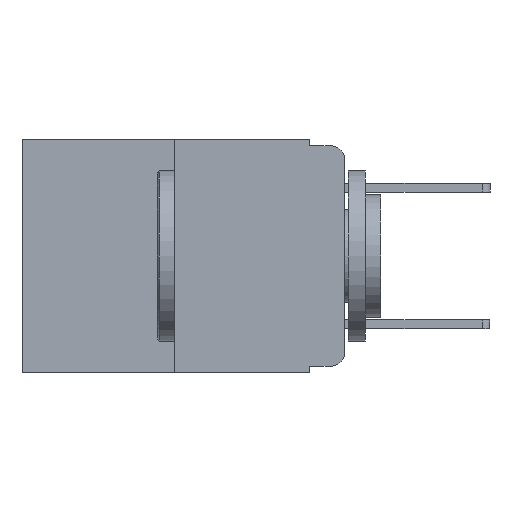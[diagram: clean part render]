
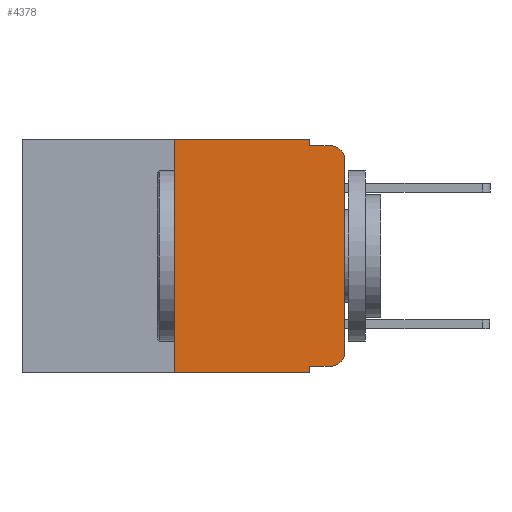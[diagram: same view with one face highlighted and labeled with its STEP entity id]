
A CAD part, left-side view. The second image highlights one B-rep face of the part: STEP entity #4378.
In plain terms, the highlighted planar face has unit normal (-1, 0, 0).
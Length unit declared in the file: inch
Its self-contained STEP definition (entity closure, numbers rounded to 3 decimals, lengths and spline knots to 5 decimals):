
#37 = DIRECTION ( 'NONE',  ( 0., 0., -1. ) ) ;
#82 = ORIENTED_EDGE ( 'NONE', *, *, #7105, .T. ) ;
#223 = LINE ( 'NONE', #6069, #14156 ) ;
#320 = ORIENTED_EDGE ( 'NONE', *, *, #5333, .T. ) ;
#467 = ORIENTED_EDGE ( 'NONE', *, *, #9116, .T. ) ;
#565 = CARTESIAN_POINT ( 'NONE',  ( 0., 0.25, 0. ) ) ;
#1006 = DIRECTION ( 'NONE',  ( 0., -1., 0. ) ) ;
#1042 = DIRECTION ( 'NONE',  ( -1., 0., 0. ) ) ;
#1183 = FACE_OUTER_BOUND ( 'NONE', #17274, .T. ) ;
#1444 = VECTOR ( 'NONE', #16356, 39.37008 ) ;
#1586 = CARTESIAN_POINT ( 'NONE',  ( 0., 0.25, 0. ) ) ;
#1604 = ORIENTED_EDGE ( 'NONE', *, *, #12360, .F. ) ;
#1745 = VERTEX_POINT ( 'NONE', #8723 ) ;
#1826 = CIRCLE ( 'NONE', #4819, 0.02 ) ;
#2852 = LINE ( 'NONE', #10554, #6090 ) ;
#3001 = DIRECTION ( 'NONE',  ( -1., 0., 0. ) ) ;
#3358 = CARTESIAN_POINT ( 'NONE',  ( 0., 0.051, -0.333 ) ) ;
#3367 = CARTESIAN_POINT ( 'NONE',  ( 0., 0.25, -0.343 ) ) ;
#3584 = LINE ( 'NONE', #8337, #10679 ) ;
#4138 = CARTESIAN_POINT ( 'NONE',  ( 0., 0., -0.313 ) ) ;
#4378 = ADVANCED_FACE ( 'NONE', ( #1183 ), #14794, .F. ) ;
#4601 = VECTOR ( 'NONE', #8008, 39.37008 ) ;
#4819 = AXIS2_PLACEMENT_3D ( 'NONE', #11004, #3001, #12320 ) ;
#4850 = VERTEX_POINT ( 'NONE', #4138 ) ;
#5333 = EDGE_CURVE ( 'NONE', #1745, #4850, #1826, .T. ) ;
#5754 = DIRECTION ( 'NONE',  ( 0., 0., -1. ) ) ;
#5773 = ORIENTED_EDGE ( 'NONE', *, *, #11507, .F. ) ;
#5962 = VERTEX_POINT ( 'NONE', #12768 ) ;
#6069 = CARTESIAN_POINT ( 'NONE',  ( 0., 0.051, -0.333 ) ) ;
#6090 = VECTOR ( 'NONE', #15634, 39.37008 ) ;
#6139 = AXIS2_PLACEMENT_3D ( 'NONE', #9271, #1042, #10580 ) ;
#6631 = CARTESIAN_POINT ( 'NONE',  ( 0., 0.473, -0.343 ) ) ;
#6642 = CARTESIAN_POINT ( 'NONE',  ( 0., 0.051, 0. ) ) ;
#6813 = ORIENTED_EDGE ( 'NONE', *, *, #13216, .T. ) ;
#7105 = EDGE_CURVE ( 'NONE', #8234, #1745, #223, .T. ) ;
#7945 = CARTESIAN_POINT ( 'NONE',  ( 0., 0.051, -0.01 ) ) ;
#7986 = VERTEX_POINT ( 'NONE', #9239 ) ;
#8003 = EDGE_CURVE ( 'NONE', #8234, #7986, #8868, .T. ) ;
#8008 = DIRECTION ( 'NONE',  ( 0., 0., 1. ) ) ;
#8163 = VERTEX_POINT ( 'NONE', #8577 ) ;
#8234 = VERTEX_POINT ( 'NONE', #3358 ) ;
#8262 = VERTEX_POINT ( 'NONE', #10106 ) ;
#8337 = CARTESIAN_POINT ( 'NONE',  ( 0., 0.051, 0. ) ) ;
#8548 = LINE ( 'NONE', #14459, #4601 ) ;
#8577 = CARTESIAN_POINT ( 'NONE',  ( 0., 0., -0.03 ) ) ;
#8582 = CARTESIAN_POINT ( 'NONE',  ( 0., 0.473, 0. ) ) ;
#8723 = CARTESIAN_POINT ( 'NONE',  ( 0., 0.02, -0.333 ) ) ;
#8868 = LINE ( 'NONE', #6642, #14911 ) ;
#8897 = EDGE_CURVE ( 'NONE', #13844, #16127, #11465, .T. ) ;
#9104 = ORIENTED_EDGE ( 'NONE', *, *, #8003, .F. ) ;
#9116 = EDGE_CURVE ( 'NONE', #13844, #7986, #12461, .T. ) ;
#9239 = CARTESIAN_POINT ( 'NONE',  ( 0., 0.051, -0.343 ) ) ;
#9271 = CARTESIAN_POINT ( 'NONE',  ( 0., 0.02, -0.03 ) ) ;
#9690 = CARTESIAN_POINT ( 'NONE',  ( 0., 0.473, 0. ) ) ;
#10106 = CARTESIAN_POINT ( 'NONE',  ( 0., 0.02, -0.01 ) ) ;
#10171 = DIRECTION ( 'NONE',  ( 0., 0., 1. ) ) ;
#10539 = ORIENTED_EDGE ( 'NONE', *, *, #8897, .F. ) ;
#10554 = CARTESIAN_POINT ( 'NONE',  ( 0., 0.051, -0.01 ) ) ;
#10580 = DIRECTION ( 'NONE',  ( 0., 0., -1. ) ) ;
#10608 = DIRECTION ( 'NONE',  ( 0., 0., -1. ) ) ;
#10679 = VECTOR ( 'NONE', #37, 39.37008 ) ;
#11004 = CARTESIAN_POINT ( 'NONE',  ( 0., 0.02, -0.313 ) ) ;
#11103 = AXIS2_PLACEMENT_3D ( 'NONE', #9690, #13579, #5754 ) ;
#11465 = LINE ( 'NONE', #565, #15284 ) ;
#11507 = EDGE_CURVE ( 'NONE', #5962, #14874, #3584, .T. ) ;
#11665 = VECTOR ( 'NONE', #1006, 39.37008 ) ;
#12018 = CIRCLE ( 'NONE', #6139, 0.02 ) ;
#12194 = LINE ( 'NONE', #8582, #1444 ) ;
#12320 = DIRECTION ( 'NONE',  ( 0., 0., -1. ) ) ;
#12360 = EDGE_CURVE ( 'NONE', #14874, #8262, #2852, .T. ) ;
#12461 = LINE ( 'NONE', #6631, #11665 ) ;
#12768 = CARTESIAN_POINT ( 'NONE',  ( 0., 0.051, 0. ) ) ;
#12781 = DIRECTION ( 'NONE',  ( 0., -1., 0. ) ) ;
#13216 = EDGE_CURVE ( 'NONE', #8163, #8262, #12018, .T. ) ;
#13549 = ORIENTED_EDGE ( 'NONE', *, *, #15604, .F. ) ;
#13579 = DIRECTION ( 'NONE',  ( 1., 0., 0. ) ) ;
#13844 = VERTEX_POINT ( 'NONE', #3367 ) ;
#14156 = VECTOR ( 'NONE', #12781, 39.37008 ) ;
#14459 = CARTESIAN_POINT ( 'NONE',  ( 0., 0., 0. ) ) ;
#14794 = PLANE ( 'NONE',  #11103 ) ;
#14874 = VERTEX_POINT ( 'NONE', #7945 ) ;
#14911 = VECTOR ( 'NONE', #10608, 39.37008 ) ;
#14939 = EDGE_CURVE ( 'NONE', #4850, #8163, #8548, .T. ) ;
#15284 = VECTOR ( 'NONE', #10171, 39.37008 ) ;
#15604 = EDGE_CURVE ( 'NONE', #16127, #5962, #12194, .T. ) ;
#15634 = DIRECTION ( 'NONE',  ( 0., -1., 0. ) ) ;
#16127 = VERTEX_POINT ( 'NONE', #1586 ) ;
#16312 = ORIENTED_EDGE ( 'NONE', *, *, #14939, .T. ) ;
#16356 = DIRECTION ( 'NONE',  ( 0., -1., 0. ) ) ;
#17274 = EDGE_LOOP ( 'NONE', ( #16312, #6813, #1604, #5773, #13549, #10539, #467, #9104, #82, #320 ) ) ;
